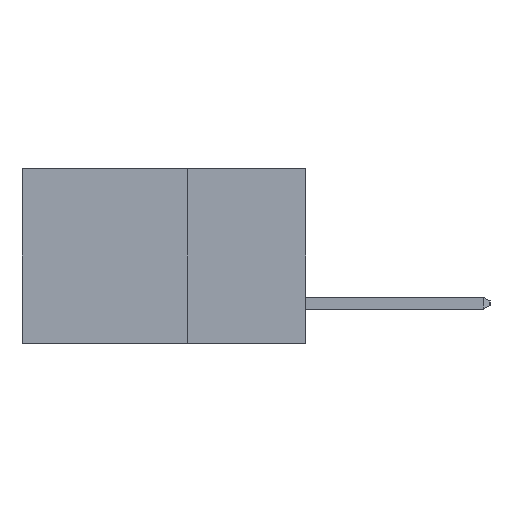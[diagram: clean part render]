
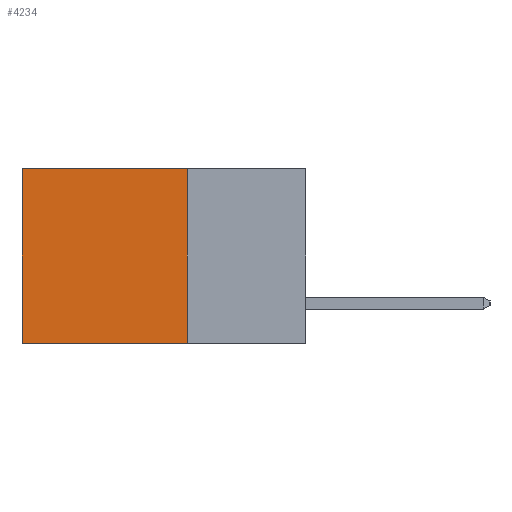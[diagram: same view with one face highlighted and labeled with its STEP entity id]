
A CAD part, left-side view. The second image highlights one B-rep face of the part: STEP entity #4234.
In plain terms, the highlighted planar face has unit normal (-1, 0, 0).
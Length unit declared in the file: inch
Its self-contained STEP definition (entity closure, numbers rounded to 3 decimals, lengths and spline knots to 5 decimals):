
#245 = CARTESIAN_POINT ( 'NONE',  ( 0.298, 0.6, 0. ) ) ;
#504 = VERTEX_POINT ( 'NONE', #245 ) ;
#879 = LINE ( 'NONE', #2313, #11231 ) ;
#1258 = EDGE_CURVE ( 'NONE', #12688, #7067, #2595, .T. ) ;
#1545 = ORIENTED_EDGE ( 'NONE', *, *, #1258, .F. ) ;
#1660 = FACE_OUTER_BOUND ( 'NONE', #1728, .T. ) ;
#1728 = EDGE_LOOP ( 'NONE', ( #11778, #1545, #12048, #9894 ) ) ;
#1966 = CARTESIAN_POINT ( 'NONE',  ( 0.298, 0.25, -0.37 ) ) ;
#2313 = CARTESIAN_POINT ( 'NONE',  ( 0.298, 0.6, 0. ) ) ;
#2595 = LINE ( 'NONE', #6791, #7979 ) ;
#2768 = AXIS2_PLACEMENT_3D ( 'NONE', #10609, #8069, #8010 ) ;
#3276 = EDGE_CURVE ( 'NONE', #4237, #12688, #6013, .T. ) ;
#4234 = ADVANCED_FACE ( 'NONE', ( #1660 ), #10591, .F. ) ;
#4237 = VERTEX_POINT ( 'NONE', #8095 ) ;
#6013 = LINE ( 'NONE', #10351, #10920 ) ;
#6129 = DIRECTION ( 'NONE',  ( 0., 1., 0. ) ) ;
#6489 = EDGE_CURVE ( 'NONE', #504, #7067, #879, .T. ) ;
#6698 = VECTOR ( 'NONE', #9195, 39.37008 ) ;
#6791 = CARTESIAN_POINT ( 'NONE',  ( 0.298, 0.25, -0.37 ) ) ;
#7031 = LINE ( 'NONE', #8215, #6698 ) ;
#7067 = VERTEX_POINT ( 'NONE', #8277 ) ;
#7874 = DIRECTION ( 'NONE',  ( 0., 0., -1. ) ) ;
#7979 = VECTOR ( 'NONE', #6129, 39.37008 ) ;
#8010 = DIRECTION ( 'NONE',  ( 0., 0., -1. ) ) ;
#8069 = DIRECTION ( 'NONE',  ( 1., 0., 0. ) ) ;
#8095 = CARTESIAN_POINT ( 'NONE',  ( 0.298, 0.25, 0. ) ) ;
#8215 = CARTESIAN_POINT ( 'NONE',  ( 0.298, 0.25, 0. ) ) ;
#8277 = CARTESIAN_POINT ( 'NONE',  ( 0.298, 0.6, -0.37 ) ) ;
#9195 = DIRECTION ( 'NONE',  ( 0., 1., 0. ) ) ;
#9894 = ORIENTED_EDGE ( 'NONE', *, *, #10352, .T. ) ;
#10351 = CARTESIAN_POINT ( 'NONE',  ( 0.298, 0.25, 0. ) ) ;
#10352 = EDGE_CURVE ( 'NONE', #4237, #504, #7031, .T. ) ;
#10388 = DIRECTION ( 'NONE',  ( 0., 0., -1. ) ) ;
#10591 = PLANE ( 'NONE',  #2768 ) ;
#10609 = CARTESIAN_POINT ( 'NONE',  ( 0.298, 0.25, 0. ) ) ;
#10920 = VECTOR ( 'NONE', #10388, 39.37008 ) ;
#11231 = VECTOR ( 'NONE', #7874, 39.37008 ) ;
#11778 = ORIENTED_EDGE ( 'NONE', *, *, #6489, .T. ) ;
#12048 = ORIENTED_EDGE ( 'NONE', *, *, #3276, .F. ) ;
#12688 = VERTEX_POINT ( 'NONE', #1966 ) ;
